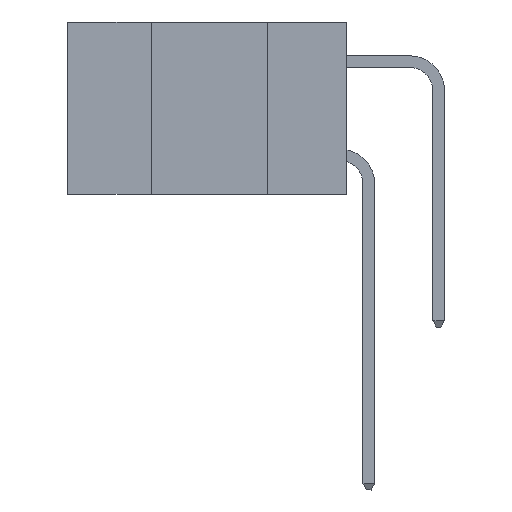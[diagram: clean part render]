
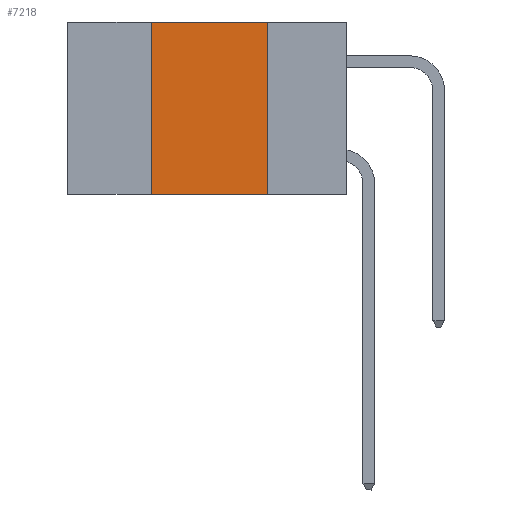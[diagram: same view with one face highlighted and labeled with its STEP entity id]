
A CAD part, left-side view. The second image highlights one B-rep face of the part: STEP entity #7218.
In plain terms, the highlighted planar face has unit normal (-1, 0, 0).
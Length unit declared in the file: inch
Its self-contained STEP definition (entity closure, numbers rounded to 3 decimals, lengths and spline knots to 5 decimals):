
#57 = DIRECTION ( 'NONE',  ( 0., -1., 0. ) ) ;
#62 = VECTOR ( 'NONE', #14977, 39.37008 ) ;
#259 = CARTESIAN_POINT ( 'NONE',  ( 0., 0.6, 0. ) ) ;
#463 = CARTESIAN_POINT ( 'NONE',  ( 0., 0.6, 0. ) ) ;
#2698 = LINE ( 'NONE', #463, #62 ) ;
#2736 = AXIS2_PLACEMENT_3D ( 'NONE', #259, #5025, #12092 ) ;
#2898 = CARTESIAN_POINT ( 'NONE',  ( 0., 0.42, 0. ) ) ;
#3899 = EDGE_CURVE ( 'NONE', #4482, #9034, #14574, .T. ) ;
#4482 = VERTEX_POINT ( 'NONE', #7514 ) ;
#5025 = DIRECTION ( 'NONE',  ( 1., 0., 0. ) ) ;
#5607 = EDGE_LOOP ( 'NONE', ( #9501, #9675, #13908, #7601 ) ) ;
#6165 = VECTOR ( 'NONE', #57, 39.37008 ) ;
#6392 = VECTOR ( 'NONE', #11729, 39.37008 ) ;
#6726 = LINE ( 'NONE', #14099, #6392 ) ;
#7122 = CARTESIAN_POINT ( 'NONE',  ( 0., 0.17, 0. ) ) ;
#7167 = VECTOR ( 'NONE', #9883, 39.37008 ) ;
#7218 = ADVANCED_FACE ( 'NONE', ( #7582 ), #12168, .F. ) ;
#7514 = CARTESIAN_POINT ( 'NONE',  ( 0., 0.42, -0.37 ) ) ;
#7582 = FACE_OUTER_BOUND ( 'NONE', #5607, .T. ) ;
#7601 = ORIENTED_EDGE ( 'NONE', *, *, #3899, .T. ) ;
#8070 = VERTEX_POINT ( 'NONE', #11235 ) ;
#8989 = CARTESIAN_POINT ( 'NONE',  ( 0., 0.17, -0.37 ) ) ;
#9034 = VERTEX_POINT ( 'NONE', #8989 ) ;
#9501 = ORIENTED_EDGE ( 'NONE', *, *, #12289, .F. ) ;
#9675 = ORIENTED_EDGE ( 'NONE', *, *, #12180, .F. ) ;
#9883 = DIRECTION ( 'NONE',  ( 0., 0., 1. ) ) ;
#11235 = CARTESIAN_POINT ( 'NONE',  ( 0., 0.42, 0. ) ) ;
#11729 = DIRECTION ( 'NONE',  ( 0., 0., -1. ) ) ;
#12092 = DIRECTION ( 'NONE',  ( 0., 0., -1. ) ) ;
#12168 = PLANE ( 'NONE',  #2736 ) ;
#12180 = EDGE_CURVE ( 'NONE', #8070, #15643, #2698, .T. ) ;
#12289 = EDGE_CURVE ( 'NONE', #15643, #9034, #6726, .T. ) ;
#13067 = CARTESIAN_POINT ( 'NONE',  ( 0., 0.6, -0.37 ) ) ;
#13746 = LINE ( 'NONE', #2898, #7167 ) ;
#13908 = ORIENTED_EDGE ( 'NONE', *, *, #14441, .F. ) ;
#14099 = CARTESIAN_POINT ( 'NONE',  ( 0., 0.17, 0. ) ) ;
#14441 = EDGE_CURVE ( 'NONE', #4482, #8070, #13746, .T. ) ;
#14574 = LINE ( 'NONE', #13067, #6165 ) ;
#14977 = DIRECTION ( 'NONE',  ( 0., -1., 0. ) ) ;
#15643 = VERTEX_POINT ( 'NONE', #7122 ) ;
